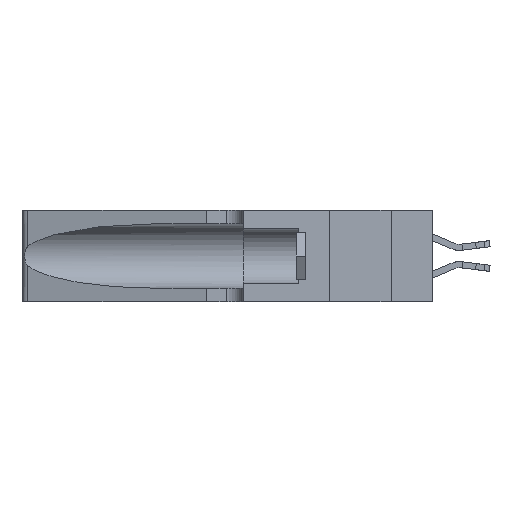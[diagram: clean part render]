
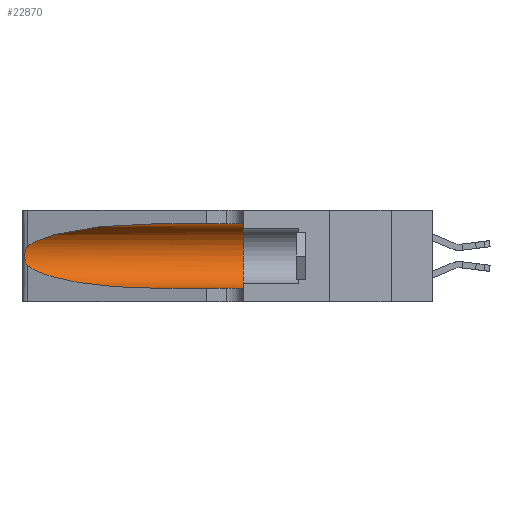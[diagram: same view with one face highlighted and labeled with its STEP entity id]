
A CAD part, left-side view. The second image highlights one B-rep face of the part: STEP entity #22870.
In plain terms, the highlighted cylindrical face has radius 3.308 mm (diameter 6.617 mm), a partial arc.
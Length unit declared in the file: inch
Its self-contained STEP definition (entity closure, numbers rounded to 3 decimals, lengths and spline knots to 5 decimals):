
#72 = CARTESIAN_POINT ( 'NONE',  ( 0.25487, 1.22718, 0.14631 ) ) ;
#611 =( BOUNDED_CURVE ( )  B_SPLINE_CURVE ( 3, ( #7125, #9042, #24020, #12893 ),
 .UNSPECIFIED., .F., .F. ) 
 B_SPLINE_CURVE_WITH_KNOTS ( ( 4, 4 ),
 ( 1.5708, 2.84003 ),
 .UNSPECIFIED. ) 
 CURVE ( )  GEOMETRIC_REPRESENTATION_ITEM ( )  RATIONAL_B_SPLINE_CURVE ( ( 1., 0.87, 0.87, 1. ) ) 
 REPRESENTATION_ITEM ( '' )  );
#686 = CARTESIAN_POINT ( 'NONE',  ( 0.1305, 0.35, 0.31525 ) ) ;
#760 = CARTESIAN_POINT ( 'NONE',  ( 0.1305, 1.61858, 0.185 ) ) ;
#1399 = ORIENTED_EDGE ( 'NONE', *, *, #8776, .T. ) ;
#1710 =( BOUNDED_CURVE ( )  B_SPLINE_CURVE ( 3, ( #72, #11636, #15420, #4027 ),
 .UNSPECIFIED., .F., .F. ) 
 B_SPLINE_CURVE_WITH_KNOTS ( ( 4, 4 ),
 ( 3.44316, 4.71239 ),
 .UNSPECIFIED. ) 
 CURVE ( )  GEOMETRIC_REPRESENTATION_ITEM ( )  RATIONAL_B_SPLINE_CURVE ( ( 1., 0.87, 0.87, 1. ) ) 
 REPRESENTATION_ITEM ( '' )  );
#1745 = CARTESIAN_POINT ( 'NONE',  ( 0.26017, 1.23833, 0.17102 ) ) ;
#2846 = CARTESIAN_POINT ( 'NONE',  ( 0.1305, 1.61858, 0.31525 ) ) ;
#2898 = VERTEX_POINT ( 'NONE', #7211 ) ;
#3248 = CIRCLE ( 'NONE', #24100, 0.13025 ) ;
#3689 = CARTESIAN_POINT ( 'NONE',  ( 0.25789, 1.23486, 0.15765 ) ) ;
#3927 = EDGE_CURVE ( 'NONE', #2898, #24545, #1710, .T. ) ;
#4027 = CARTESIAN_POINT ( 'NONE',  ( 0.1305, 0.72297, 0.05475 ) ) ;
#4891 = ORIENTED_EDGE ( 'NONE', *, *, #3927, .T. ) ;
#5267 = DIRECTION ( 'NONE',  ( 0., 1., 0. ) ) ;
#5569 = CARTESIAN_POINT ( 'NONE',  ( 0.25487, 1.22718, 0.22369 ) ) ;
#5650 = CARTESIAN_POINT ( 'NONE',  ( 0.25555, 1.22993, 0.14849 ) ) ;
#6151 = VERTEX_POINT ( 'NONE', #8706 ) ;
#6749 = ORIENTED_EDGE ( 'NONE', *, *, #16634, .F. ) ;
#7125 = CARTESIAN_POINT ( 'NONE',  ( 0.1305, 0.72297, 0.31525 ) ) ;
#7211 = CARTESIAN_POINT ( 'NONE',  ( 0.25487, 1.22718, 0.14631 ) ) ;
#7349 = EDGE_CURVE ( 'NONE', #24545, #6151, #19158, .T. ) ;
#8127 = CYLINDRICAL_SURFACE ( 'NONE', #15413, 0.13025 ) ;
#8546 = VERTEX_POINT ( 'NONE', #14048 ) ;
#8706 = CARTESIAN_POINT ( 'NONE',  ( 0.1305, 0.35, 0.05475 ) ) ;
#8776 = EDGE_CURVE ( 'NONE', #11048, #8546, #611, .T. ) ;
#9042 = CARTESIAN_POINT ( 'NONE',  ( 0.18966, 0.96281, 0.31525 ) ) ;
#9408 = CARTESIAN_POINT ( 'NONE',  ( 0.25787, 1.23484, 0.2124 ) ) ;
#10078 = LINE ( 'NONE', #2846, #19481 ) ;
#11048 = VERTEX_POINT ( 'NONE', #16656 ) ;
#11331 = CARTESIAN_POINT ( 'NONE',  ( 0.26018, 1.23835, 0.19895 ) ) ;
#11636 = CARTESIAN_POINT ( 'NONE',  ( 0.2373, 1.15595, 0.08982 ) ) ;
#12893 = CARTESIAN_POINT ( 'NONE',  ( 0.25487, 1.22718, 0.22369 ) ) ;
#12900 = EDGE_LOOP ( 'NONE', ( #1399, #13287, #4891, #23658, #14546, #6749 ) ) ;
#13242 = CARTESIAN_POINT ( 'NONE',  ( 0.26075, 1.23896, 0.178 ) ) ;
#13287 = ORIENTED_EDGE ( 'NONE', *, *, #18258, .T. ) ;
#13324 = CARTESIAN_POINT ( 'NONE',  ( 0.1305, 0.72297, 0.05475 ) ) ;
#13701 = B_SPLINE_CURVE_WITH_KNOTS ( 'NONE', 3,
 ( #5569, #18800, #20642, #9408, #22522, #11331, #24378, #13242, #1745, #15110, #3689, #17018, #5650, #18880 ),
 .UNSPECIFIED., .F., .F.,
 ( 4, 2, 2, 2, 2, 2, 4 ),
 ( 0., 0.00027, 0.00053, 0.00107, 0.0016, 0.00187, 0.00214 ),
 .UNSPECIFIED. ) ;
#14048 = CARTESIAN_POINT ( 'NONE',  ( 0.25487, 1.22718, 0.22369 ) ) ;
#14195 = DIRECTION ( 'NONE',  ( 0., -1., 0. ) ) ;
#14546 = ORIENTED_EDGE ( 'NONE', *, *, #20393, .F. ) ;
#14784 = VECTOR ( 'NONE', #17792, 39.37008 ) ;
#15110 = CARTESIAN_POINT ( 'NONE',  ( 0.25856, 1.23593, 0.16098 ) ) ;
#15413 = AXIS2_PLACEMENT_3D ( 'NONE', #760, #14195, #16076 ) ;
#15420 = CARTESIAN_POINT ( 'NONE',  ( 0.18966, 0.96281, 0.05475 ) ) ;
#16076 = DIRECTION ( 'NONE',  ( 0., 0., -1. ) ) ;
#16193 = DIRECTION ( 'NONE',  ( 0., -1., 0. ) ) ;
#16634 = EDGE_CURVE ( 'NONE', #11048, #19657, #10078, .T. ) ;
#16636 = CARTESIAN_POINT ( 'NONE',  ( 0.1305, 0.35, 0.185 ) ) ;
#16656 = CARTESIAN_POINT ( 'NONE',  ( 0.1305, 0.72297, 0.31525 ) ) ;
#17018 = CARTESIAN_POINT ( 'NONE',  ( 0.25639, 1.23186, 0.15144 ) ) ;
#17792 = DIRECTION ( 'NONE',  ( 0., -1., 0. ) ) ;
#17873 = CARTESIAN_POINT ( 'NONE',  ( 0.1305, 1.61858, 0.05475 ) ) ;
#18258 = EDGE_CURVE ( 'NONE', #8546, #2898, #13701, .T. ) ;
#18506 = DIRECTION ( 'NONE',  ( 0., 0., 1. ) ) ;
#18776 = FACE_OUTER_BOUND ( 'NONE', #12900, .T. ) ;
#18800 = CARTESIAN_POINT ( 'NONE',  ( 0.25555, 1.22994, 0.2215 ) ) ;
#18880 = CARTESIAN_POINT ( 'NONE',  ( 0.25487, 1.22718, 0.14631 ) ) ;
#19158 = LINE ( 'NONE', #17873, #14784 ) ;
#19481 = VECTOR ( 'NONE', #16193, 39.37008 ) ;
#19657 = VERTEX_POINT ( 'NONE', #686 ) ;
#20393 = EDGE_CURVE ( 'NONE', #19657, #6151, #3248, .T. ) ;
#20642 = CARTESIAN_POINT ( 'NONE',  ( 0.25639, 1.23184, 0.21858 ) ) ;
#22522 = CARTESIAN_POINT ( 'NONE',  ( 0.25854, 1.2359, 0.20912 ) ) ;
#22870 = ADVANCED_FACE ( 'NONE', ( #18776 ), #8127, .F. ) ;
#23658 = ORIENTED_EDGE ( 'NONE', *, *, #7349, .T. ) ;
#24020 = CARTESIAN_POINT ( 'NONE',  ( 0.2373, 1.15595, 0.28018 ) ) ;
#24100 = AXIS2_PLACEMENT_3D ( 'NONE', #16636, #5267, #18506 ) ;
#24378 = CARTESIAN_POINT ( 'NONE',  ( 0.26075, 1.23896, 0.19203 ) ) ;
#24545 = VERTEX_POINT ( 'NONE', #13324 ) ;
